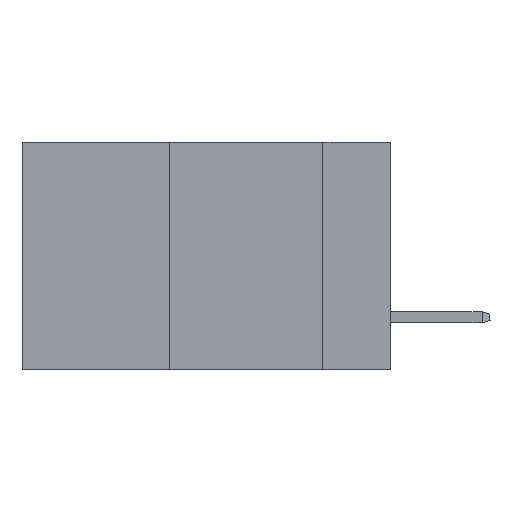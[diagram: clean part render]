
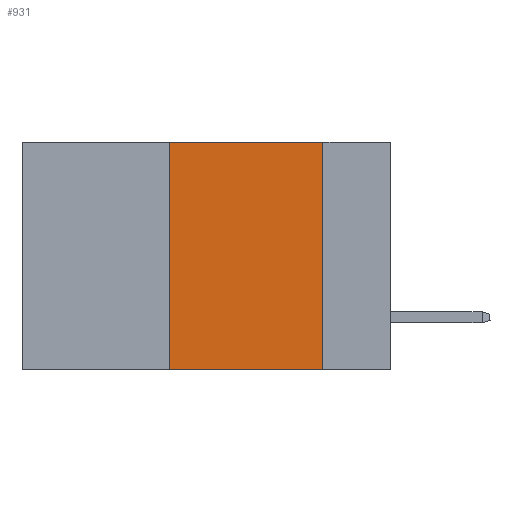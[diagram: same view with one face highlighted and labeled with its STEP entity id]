
A CAD part, left-side view. The second image highlights one B-rep face of the part: STEP entity #931.
In plain terms, the highlighted planar face has unit normal (-1, 0, 0).
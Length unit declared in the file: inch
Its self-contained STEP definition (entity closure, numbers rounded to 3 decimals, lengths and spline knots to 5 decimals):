
#931 = ADVANCED_FACE ( 'NONE', ( #15156 ), #17014, .F. ) ;
#1311 = EDGE_LOOP ( 'NONE', ( #12263, #17275, #8121, #15541 ) ) ;
#1753 = VECTOR ( 'NONE', #5438, 39.37008 ) ;
#1912 = VERTEX_POINT ( 'NONE', #18681 ) ;
#2348 = LINE ( 'NONE', #5529, #1753 ) ;
#2385 = AXIS2_PLACEMENT_3D ( 'NONE', #10464, #18059, #18230 ) ;
#2423 = VECTOR ( 'NONE', #18258, 39.37008 ) ;
#3407 = VERTEX_POINT ( 'NONE', #14881 ) ;
#3930 = CARTESIAN_POINT ( 'NONE',  ( 0., 0.11, 0. ) ) ;
#5438 = DIRECTION ( 'NONE',  ( 0., 0., -1. ) ) ;
#5529 = CARTESIAN_POINT ( 'NONE',  ( 0., 0.11, 0. ) ) ;
#6157 = DIRECTION ( 'NONE',  ( 0., 0., 1. ) ) ;
#7448 = CARTESIAN_POINT ( 'NONE',  ( 0., 0.36, 0. ) ) ;
#8121 = ORIENTED_EDGE ( 'NONE', *, *, #22202, .F. ) ;
#8129 = VECTOR ( 'NONE', #6157, 39.37008 ) ;
#8234 = CARTESIAN_POINT ( 'NONE',  ( 0., 0.36, 0. ) ) ;
#9159 = VERTEX_POINT ( 'NONE', #7448 ) ;
#9903 = CARTESIAN_POINT ( 'NONE',  ( 0., 0.6, 0. ) ) ;
#9999 = LINE ( 'NONE', #9903, #19672 ) ;
#10464 = CARTESIAN_POINT ( 'NONE',  ( 0., 0.6, 0. ) ) ;
#12096 = LINE ( 'NONE', #8234, #8129 ) ;
#12263 = ORIENTED_EDGE ( 'NONE', *, *, #14621, .F. ) ;
#13237 = EDGE_CURVE ( 'NONE', #9159, #16737, #9999, .T. ) ;
#13303 = EDGE_CURVE ( 'NONE', #3407, #1912, #19402, .T. ) ;
#14621 = EDGE_CURVE ( 'NONE', #16737, #1912, #2348, .T. ) ;
#14881 = CARTESIAN_POINT ( 'NONE',  ( 0., 0.36, -0.37 ) ) ;
#15156 = FACE_OUTER_BOUND ( 'NONE', #1311, .T. ) ;
#15541 = ORIENTED_EDGE ( 'NONE', *, *, #13303, .T. ) ;
#16737 = VERTEX_POINT ( 'NONE', #3930 ) ;
#17014 = PLANE ( 'NONE',  #2385 ) ;
#17275 = ORIENTED_EDGE ( 'NONE', *, *, #13237, .F. ) ;
#17932 = CARTESIAN_POINT ( 'NONE',  ( 0., 0.6, -0.37 ) ) ;
#18059 = DIRECTION ( 'NONE',  ( 1., 0., 0. ) ) ;
#18230 = DIRECTION ( 'NONE',  ( 0., 0., -1. ) ) ;
#18258 = DIRECTION ( 'NONE',  ( 0., -1., 0. ) ) ;
#18681 = CARTESIAN_POINT ( 'NONE',  ( 0., 0.11, -0.37 ) ) ;
#19402 = LINE ( 'NONE', #17932, #2423 ) ;
#19672 = VECTOR ( 'NONE', #19763, 39.37008 ) ;
#19763 = DIRECTION ( 'NONE',  ( 0., -1., 0. ) ) ;
#22202 = EDGE_CURVE ( 'NONE', #3407, #9159, #12096, .T. ) ;
